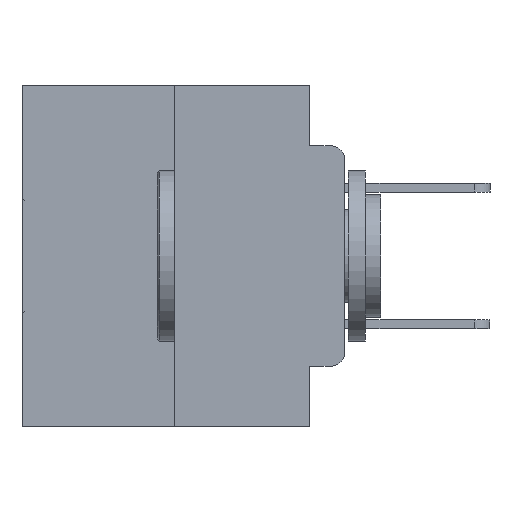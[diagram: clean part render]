
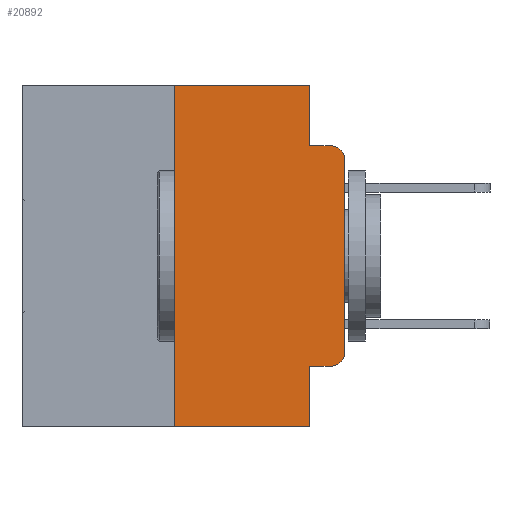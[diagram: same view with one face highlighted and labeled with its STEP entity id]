
A CAD part, left-side view. The second image highlights one B-rep face of the part: STEP entity #20892.
In plain terms, the highlighted planar face has unit normal (-1, 0, 0).
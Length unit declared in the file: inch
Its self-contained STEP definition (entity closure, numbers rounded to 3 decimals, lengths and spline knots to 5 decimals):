
#595 = DIRECTION ( 'NONE',  ( 1., 0., 0. ) ) ;
#1044 = DIRECTION ( 'NONE',  ( 0., -1., 0. ) ) ;
#1939 = CARTESIAN_POINT ( 'NONE',  ( 0., 0.02, -0.1085 ) ) ;
#2508 = CARTESIAN_POINT ( 'NONE',  ( 0., 0.02, -0.3915 ) ) ;
#2580 = VECTOR ( 'NONE', #24060, 39.37008 ) ;
#2930 = EDGE_CURVE ( 'NONE', #18389, #24524, #11092, .T. ) ;
#3539 = CARTESIAN_POINT ( 'NONE',  ( 0., 0.473, 0. ) ) ;
#4456 = DIRECTION ( 'NONE',  ( 0., 0., -1. ) ) ;
#4964 = DIRECTION ( 'NONE',  ( 0., 0., -1. ) ) ;
#5134 = LINE ( 'NONE', #9385, #28426 ) ;
#5541 = LINE ( 'NONE', #19295, #10883 ) ;
#6057 = CARTESIAN_POINT ( 'NONE',  ( 0., 0.051, 0. ) ) ;
#7796 = FACE_OUTER_BOUND ( 'NONE', #23813, .T. ) ;
#8204 = CARTESIAN_POINT ( 'NONE',  ( 0., 0.051, 0. ) ) ;
#8810 = LINE ( 'NONE', #8204, #2580 ) ;
#9167 = EDGE_CURVE ( 'NONE', #24524, #11634, #20567, .T. ) ;
#9187 = VERTEX_POINT ( 'NONE', #20807 ) ;
#9266 = DIRECTION ( 'NONE',  ( 0., 0., 1. ) ) ;
#9385 = CARTESIAN_POINT ( 'NONE',  ( 0., 0.051, -0.0885 ) ) ;
#9831 = CARTESIAN_POINT ( 'NONE',  ( 0., 0.473, -0.5 ) ) ;
#9969 = PLANE ( 'NONE',  #22936 ) ;
#10069 = AXIS2_PLACEMENT_3D ( 'NONE', #2508, #18557, #4964 ) ;
#10291 = DIRECTION ( 'NONE',  ( 0., 0., -1. ) ) ;
#10688 = EDGE_CURVE ( 'NONE', #18389, #19784, #8810, .T. ) ;
#10883 = VECTOR ( 'NONE', #10291, 39.37008 ) ;
#11092 = LINE ( 'NONE', #16009, #16430 ) ;
#11634 = VERTEX_POINT ( 'NONE', #12710 ) ;
#12112 = DIRECTION ( 'NONE',  ( 0., -1., 0. ) ) ;
#12202 = EDGE_CURVE ( 'NONE', #16738, #28445, #5541, .T. ) ;
#12710 = CARTESIAN_POINT ( 'NONE',  ( 0., 0., -0.3915 ) ) ;
#12717 = CARTESIAN_POINT ( 'NONE',  ( 0., 0., 0. ) ) ;
#14487 = CARTESIAN_POINT ( 'NONE',  ( 0., 0.02, -0.0885 ) ) ;
#14918 = LINE ( 'NONE', #9831, #26124 ) ;
#16009 = CARTESIAN_POINT ( 'NONE',  ( 0., 0.051, -0.4115 ) ) ;
#16041 = CARTESIAN_POINT ( 'NONE',  ( 0., 0.25, 0. ) ) ;
#16430 = VECTOR ( 'NONE', #27872, 39.37008 ) ;
#16433 = CARTESIAN_POINT ( 'NONE',  ( 0., 0.25, 0. ) ) ;
#16738 = VERTEX_POINT ( 'NONE', #6057 ) ;
#16840 = DIRECTION ( 'NONE',  ( 0., 0., -1. ) ) ;
#17990 = EDGE_CURVE ( 'NONE', #26689, #16738, #27701, .T. ) ;
#18074 = DIRECTION ( 'NONE',  ( -1., 0., 0. ) ) ;
#18272 = EDGE_CURVE ( 'NONE', #9187, #26689, #24532, .T. ) ;
#18389 = VERTEX_POINT ( 'NONE', #20815 ) ;
#18557 = DIRECTION ( 'NONE',  ( -1., 0., 0. ) ) ;
#18569 = VECTOR ( 'NONE', #9266, 39.37008 ) ;
#18652 = CARTESIAN_POINT ( 'NONE',  ( 0., 0., -0.1085 ) ) ;
#19269 = ORIENTED_EDGE ( 'NONE', *, *, #12202, .F. ) ;
#19295 = CARTESIAN_POINT ( 'NONE',  ( 0., 0.051, 0. ) ) ;
#19560 = ORIENTED_EDGE ( 'NONE', *, *, #28745, .T. ) ;
#19614 = ORIENTED_EDGE ( 'NONE', *, *, #19792, .T. ) ;
#19784 = VERTEX_POINT ( 'NONE', #23836 ) ;
#19792 = EDGE_CURVE ( 'NONE', #11634, #21414, #20242, .T. ) ;
#19894 = ORIENTED_EDGE ( 'NONE', *, *, #17990, .F. ) ;
#20242 = LINE ( 'NONE', #12717, #25495 ) ;
#20567 = CIRCLE ( 'NONE', #10069, 0.02 ) ;
#20807 = CARTESIAN_POINT ( 'NONE',  ( 0., 0.25, -0.5 ) ) ;
#20815 = CARTESIAN_POINT ( 'NONE',  ( 0., 0.051, -0.4115 ) ) ;
#20885 = VERTEX_POINT ( 'NONE', #14487 ) ;
#20892 = ADVANCED_FACE ( 'NONE', ( #7796 ), #9969, .F. ) ;
#21031 = VECTOR ( 'NONE', #1044, 39.37008 ) ;
#21210 = CARTESIAN_POINT ( 'NONE',  ( 0., 0.473, 0. ) ) ;
#21414 = VERTEX_POINT ( 'NONE', #18652 ) ;
#21483 = ORIENTED_EDGE ( 'NONE', *, *, #24281, .F. ) ;
#22894 = DIRECTION ( 'NONE',  ( 0., -1., 0. ) ) ;
#22895 = AXIS2_PLACEMENT_3D ( 'NONE', #1939, #18074, #4456 ) ;
#22936 = AXIS2_PLACEMENT_3D ( 'NONE', #21210, #595, #16840 ) ;
#23562 = CARTESIAN_POINT ( 'NONE',  ( 0., 0.051, -0.0885 ) ) ;
#23813 = EDGE_LOOP ( 'NONE', ( #19614, #19560, #21483, #19269, #19894, #24654, #26731, #25019, #24639, #24313 ) ) ;
#23836 = CARTESIAN_POINT ( 'NONE',  ( 0., 0.051, -0.5 ) ) ;
#23931 = DIRECTION ( 'NONE',  ( 0., 0., 1. ) ) ;
#24060 = DIRECTION ( 'NONE',  ( 0., 0., -1. ) ) ;
#24281 = EDGE_CURVE ( 'NONE', #28445, #20885, #5134, .T. ) ;
#24313 = ORIENTED_EDGE ( 'NONE', *, *, #9167, .T. ) ;
#24524 = VERTEX_POINT ( 'NONE', #28256 ) ;
#24532 = LINE ( 'NONE', #16041, #18569 ) ;
#24639 = ORIENTED_EDGE ( 'NONE', *, *, #2930, .T. ) ;
#24654 = ORIENTED_EDGE ( 'NONE', *, *, #18272, .F. ) ;
#25019 = ORIENTED_EDGE ( 'NONE', *, *, #10688, .F. ) ;
#25495 = VECTOR ( 'NONE', #23931, 39.37008 ) ;
#25783 = CIRCLE ( 'NONE', #22895, 0.02 ) ;
#26124 = VECTOR ( 'NONE', #12112, 39.37008 ) ;
#26689 = VERTEX_POINT ( 'NONE', #16433 ) ;
#26731 = ORIENTED_EDGE ( 'NONE', *, *, #28949, .T. ) ;
#27701 = LINE ( 'NONE', #3539, #21031 ) ;
#27872 = DIRECTION ( 'NONE',  ( 0., -1., 0. ) ) ;
#28256 = CARTESIAN_POINT ( 'NONE',  ( 0., 0.02, -0.4115 ) ) ;
#28426 = VECTOR ( 'NONE', #22894, 39.37008 ) ;
#28445 = VERTEX_POINT ( 'NONE', #23562 ) ;
#28745 = EDGE_CURVE ( 'NONE', #21414, #20885, #25783, .T. ) ;
#28949 = EDGE_CURVE ( 'NONE', #9187, #19784, #14918, .T. ) ;
